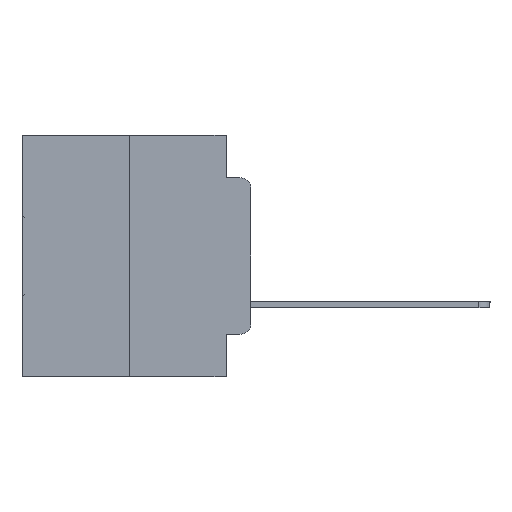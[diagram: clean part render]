
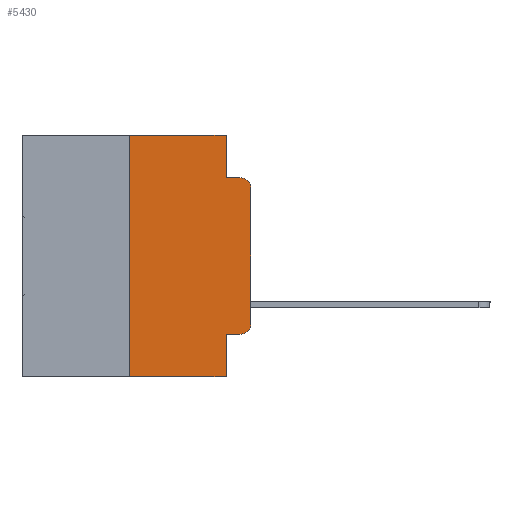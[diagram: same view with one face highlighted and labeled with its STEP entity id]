
A CAD part, left-side view. The second image highlights one B-rep face of the part: STEP entity #5430.
In plain terms, the highlighted planar face has unit normal (-1, 0, 0).
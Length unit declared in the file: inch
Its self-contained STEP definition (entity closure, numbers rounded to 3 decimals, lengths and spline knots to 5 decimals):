
#298 = CARTESIAN_POINT ( 'NONE',  ( 0., 0.25, 0. ) ) ;
#898 = CARTESIAN_POINT ( 'NONE',  ( 0., 0.051, -0.4115 ) ) ;
#1412 = VERTEX_POINT ( 'NONE', #23544 ) ;
#1690 = CARTESIAN_POINT ( 'NONE',  ( 0., 0.02, -0.4115 ) ) ;
#1803 = CARTESIAN_POINT ( 'NONE',  ( 0., 0.02, -0.3915 ) ) ;
#2306 = EDGE_CURVE ( 'NONE', #8113, #5750, #9520, .T. ) ;
#2327 = DIRECTION ( 'NONE',  ( 0., 0., -1. ) ) ;
#2359 = DIRECTION ( 'NONE',  ( 0., -1., 0. ) ) ;
#2680 = VECTOR ( 'NONE', #12125, 39.37008 ) ;
#3693 = VERTEX_POINT ( 'NONE', #298 ) ;
#3892 = DIRECTION ( 'NONE',  ( -1., 0., 0. ) ) ;
#4146 = VECTOR ( 'NONE', #2359, 39.37008 ) ;
#4218 = CARTESIAN_POINT ( 'NONE',  ( 0., 0.02, -0.0885 ) ) ;
#4715 = CARTESIAN_POINT ( 'NONE',  ( 0., 0.473, -0.5 ) ) ;
#4933 = EDGE_CURVE ( 'NONE', #25130, #5750, #18529, .T. ) ;
#5032 = LINE ( 'NONE', #14379, #27837 ) ;
#5126 = VERTEX_POINT ( 'NONE', #7703 ) ;
#5373 = EDGE_CURVE ( 'NONE', #8113, #23880, #26241, .T. ) ;
#5399 = DIRECTION ( 'NONE',  ( 0., 0., -1. ) ) ;
#5430 = ADVANCED_FACE ( 'NONE', ( #14645 ), #9434, .F. ) ;
#5436 = ORIENTED_EDGE ( 'NONE', *, *, #4933, .T. ) ;
#5750 = VERTEX_POINT ( 'NONE', #20972 ) ;
#6389 = AXIS2_PLACEMENT_3D ( 'NONE', #1803, #31080, #11465 ) ;
#6643 = ORIENTED_EDGE ( 'NONE', *, *, #5373, .T. ) ;
#6715 = AXIS2_PLACEMENT_3D ( 'NONE', #16704, #23866, #2327 ) ;
#7589 = EDGE_CURVE ( 'NONE', #20470, #1412, #21598, .T. ) ;
#7703 = CARTESIAN_POINT ( 'NONE',  ( 0., 0., -0.1085 ) ) ;
#7762 = EDGE_LOOP ( 'NONE', ( #26006, #25365, #7832, #9496, #16488, #30369, #5436, #25043, #6643, #22810 ) ) ;
#7832 = ORIENTED_EDGE ( 'NONE', *, *, #8455, .F. ) ;
#8113 = VERTEX_POINT ( 'NONE', #898 ) ;
#8160 = LINE ( 'NONE', #13704, #13048 ) ;
#8263 = EDGE_CURVE ( 'NONE', #3693, #20470, #8160, .T. ) ;
#8455 = EDGE_CURVE ( 'NONE', #1412, #18768, #29380, .T. ) ;
#9064 = VECTOR ( 'NONE', #28607, 39.37008 ) ;
#9126 = VECTOR ( 'NONE', #29531, 39.37008 ) ;
#9201 = DIRECTION ( 'NONE',  ( 0., 0., -1. ) ) ;
#9434 = PLANE ( 'NONE',  #6715 ) ;
#9496 = ORIENTED_EDGE ( 'NONE', *, *, #7589, .F. ) ;
#9520 = LINE ( 'NONE', #11430, #25031 ) ;
#10056 = EDGE_CURVE ( 'NONE', #23880, #12099, #21073, .T. ) ;
#11177 = DIRECTION ( 'NONE',  ( 0., 0., -1. ) ) ;
#11336 = DIRECTION ( 'NONE',  ( 0., -1., 0. ) ) ;
#11430 = CARTESIAN_POINT ( 'NONE',  ( 0., 0.051, 0. ) ) ;
#11465 = DIRECTION ( 'NONE',  ( 0., 0., -1. ) ) ;
#12099 = VERTEX_POINT ( 'NONE', #15543 ) ;
#12125 = DIRECTION ( 'NONE',  ( 0., -1., 0. ) ) ;
#12933 = EDGE_CURVE ( 'NONE', #12099, #5126, #24330, .T. ) ;
#13048 = VECTOR ( 'NONE', #11336, 39.37008 ) ;
#13523 = CARTESIAN_POINT ( 'NONE',  ( 0., 0.051, 0. ) ) ;
#13704 = CARTESIAN_POINT ( 'NONE',  ( 0., 0.473, 0. ) ) ;
#14362 = EDGE_CURVE ( 'NONE', #25130, #3693, #5032, .T. ) ;
#14379 = CARTESIAN_POINT ( 'NONE',  ( 0., 0.25, 0. ) ) ;
#14492 = CARTESIAN_POINT ( 'NONE',  ( 0., 0., 0. ) ) ;
#14645 = FACE_OUTER_BOUND ( 'NONE', #7762, .T. ) ;
#14993 = DIRECTION ( 'NONE',  ( 0., 0., 1. ) ) ;
#15543 = CARTESIAN_POINT ( 'NONE',  ( 0., 0., -0.3915 ) ) ;
#16488 = ORIENTED_EDGE ( 'NONE', *, *, #8263, .F. ) ;
#16704 = CARTESIAN_POINT ( 'NONE',  ( 0., 0.473, 0. ) ) ;
#16859 = CARTESIAN_POINT ( 'NONE',  ( 0., 0.051, -0.4115 ) ) ;
#17117 = CARTESIAN_POINT ( 'NONE',  ( 0., 0.051, 0. ) ) ;
#18529 = LINE ( 'NONE', #4715, #4146 ) ;
#18768 = VERTEX_POINT ( 'NONE', #4218 ) ;
#20470 = VERTEX_POINT ( 'NONE', #13523 ) ;
#20972 = CARTESIAN_POINT ( 'NONE',  ( 0., 0.051, -0.5 ) ) ;
#21073 = CIRCLE ( 'NONE', #6389, 0.02 ) ;
#21598 = LINE ( 'NONE', #17117, #28222 ) ;
#22810 = ORIENTED_EDGE ( 'NONE', *, *, #10056, .T. ) ;
#23544 = CARTESIAN_POINT ( 'NONE',  ( 0., 0.051, -0.0885 ) ) ;
#23866 = DIRECTION ( 'NONE',  ( 1., 0., 0. ) ) ;
#23880 = VERTEX_POINT ( 'NONE', #1690 ) ;
#24330 = LINE ( 'NONE', #14492, #9064 ) ;
#25031 = VECTOR ( 'NONE', #9201, 39.37008 ) ;
#25043 = ORIENTED_EDGE ( 'NONE', *, *, #2306, .F. ) ;
#25130 = VERTEX_POINT ( 'NONE', #29470 ) ;
#25365 = ORIENTED_EDGE ( 'NONE', *, *, #31158, .T. ) ;
#25381 = AXIS2_PLACEMENT_3D ( 'NONE', #25599, #3892, #11177 ) ;
#25599 = CARTESIAN_POINT ( 'NONE',  ( 0., 0.02, -0.1085 ) ) ;
#26006 = ORIENTED_EDGE ( 'NONE', *, *, #12933, .T. ) ;
#26241 = LINE ( 'NONE', #16859, #2680 ) ;
#27837 = VECTOR ( 'NONE', #14993, 39.37008 ) ;
#28222 = VECTOR ( 'NONE', #5399, 39.37008 ) ;
#28607 = DIRECTION ( 'NONE',  ( 0., 0., 1. ) ) ;
#29380 = LINE ( 'NONE', #29681, #9126 ) ;
#29433 = CIRCLE ( 'NONE', #25381, 0.02 ) ;
#29470 = CARTESIAN_POINT ( 'NONE',  ( 0., 0.25, -0.5 ) ) ;
#29531 = DIRECTION ( 'NONE',  ( 0., -1., 0. ) ) ;
#29681 = CARTESIAN_POINT ( 'NONE',  ( 0., 0.051, -0.0885 ) ) ;
#30369 = ORIENTED_EDGE ( 'NONE', *, *, #14362, .F. ) ;
#31080 = DIRECTION ( 'NONE',  ( -1., 0., 0. ) ) ;
#31158 = EDGE_CURVE ( 'NONE', #5126, #18768, #29433, .T. ) ;
